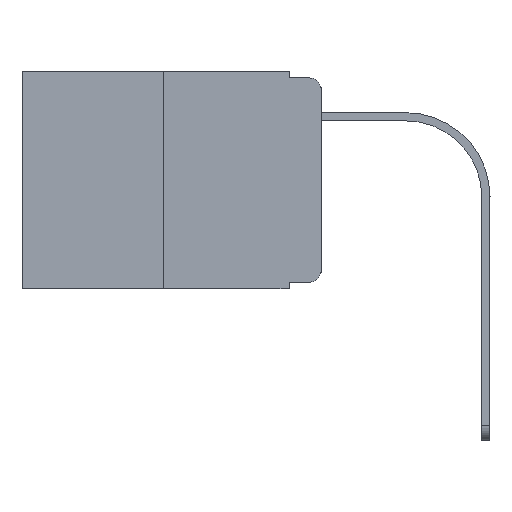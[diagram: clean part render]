
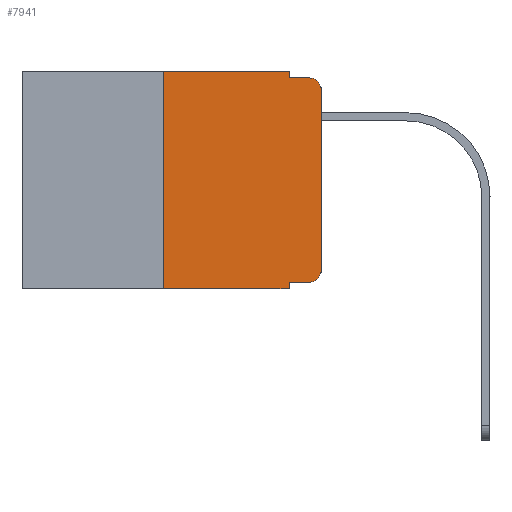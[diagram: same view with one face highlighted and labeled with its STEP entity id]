
A CAD part, left-side view. The second image highlights one B-rep face of the part: STEP entity #7941.
In plain terms, the highlighted planar face has unit normal (-1, 0, 0).
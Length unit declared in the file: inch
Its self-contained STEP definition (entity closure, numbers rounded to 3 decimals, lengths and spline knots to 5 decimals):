
#130 = VECTOR ( 'NONE', #17695, 39.37008 ) ;
#359 = PLANE ( 'NONE',  #10256 ) ;
#586 = DIRECTION ( 'NONE',  ( 0., -1., 0. ) ) ;
#771 = CIRCLE ( 'NONE', #4954, 0.02 ) ;
#1702 = VERTEX_POINT ( 'NONE', #5102 ) ;
#1730 = LINE ( 'NONE', #12129, #6146 ) ;
#1750 = EDGE_CURVE ( 'NONE', #2048, #12423, #1730, .T. ) ;
#1771 = DIRECTION ( 'NONE',  ( 1., 0., 0. ) ) ;
#1846 = VERTEX_POINT ( 'NONE', #15604 ) ;
#2048 = VERTEX_POINT ( 'NONE', #16135 ) ;
#4032 = ORIENTED_EDGE ( 'NONE', *, *, #6118, .T. ) ;
#4189 = CARTESIAN_POINT ( 'NONE',  ( 0., 0.25, -0.343 ) ) ;
#4335 = VECTOR ( 'NONE', #13827, 39.37008 ) ;
#4568 = EDGE_CURVE ( 'NONE', #15227, #15545, #4579, .T. ) ;
#4579 = LINE ( 'NONE', #11180, #130 ) ;
#4929 = ORIENTED_EDGE ( 'NONE', *, *, #4568, .F. ) ;
#4954 = AXIS2_PLACEMENT_3D ( 'NONE', #9097, #15707, #5849 ) ;
#5032 = VERTEX_POINT ( 'NONE', #9274 ) ;
#5056 = EDGE_CURVE ( 'NONE', #1702, #5032, #15770, .T. ) ;
#5102 = CARTESIAN_POINT ( 'NONE',  ( 0., 0.051, -0.333 ) ) ;
#5849 = DIRECTION ( 'NONE',  ( 0., 0., -1. ) ) ;
#6114 = DIRECTION ( 'NONE',  ( -1., 0., 0. ) ) ;
#6118 = EDGE_CURVE ( 'NONE', #1846, #15312, #16435, .T. ) ;
#6146 = VECTOR ( 'NONE', #13327, 39.37008 ) ;
#6446 = ORIENTED_EDGE ( 'NONE', *, *, #16430, .T. ) ;
#6558 = VECTOR ( 'NONE', #8209, 39.37008 ) ;
#6667 = CARTESIAN_POINT ( 'NONE',  ( 0., 0.02, -0.333 ) ) ;
#7365 = EDGE_CURVE ( 'NONE', #15545, #2048, #10957, .T. ) ;
#7546 = CARTESIAN_POINT ( 'NONE',  ( 0., 0.051, 0. ) ) ;
#7941 = ADVANCED_FACE ( 'NONE', ( #11637 ), #359, .F. ) ;
#8165 = ORIENTED_EDGE ( 'NONE', *, *, #1750, .F. ) ;
#8209 = DIRECTION ( 'NONE',  ( 0., 0., 1. ) ) ;
#8402 = DIRECTION ( 'NONE',  ( 0., 0., -1. ) ) ;
#8715 = DIRECTION ( 'NONE',  ( 0., 0., 1. ) ) ;
#9097 = CARTESIAN_POINT ( 'NONE',  ( 0., 0.02, -0.03 ) ) ;
#9264 = DIRECTION ( 'NONE',  ( 0., 0., -1. ) ) ;
#9274 = CARTESIAN_POINT ( 'NONE',  ( 0., 0.051, -0.343 ) ) ;
#9454 = ORIENTED_EDGE ( 'NONE', *, *, #19110, .T. ) ;
#10018 = CARTESIAN_POINT ( 'NONE',  ( 0., 0.473, 0. ) ) ;
#10256 = AXIS2_PLACEMENT_3D ( 'NONE', #10018, #1771, #8402 ) ;
#10433 = CARTESIAN_POINT ( 'NONE',  ( 0., 0.25, 0. ) ) ;
#10926 = AXIS2_PLACEMENT_3D ( 'NONE', #17606, #6114, #9264 ) ;
#10957 = LINE ( 'NONE', #21236, #12675 ) ;
#11180 = CARTESIAN_POINT ( 'NONE',  ( 0., 0.473, 0. ) ) ;
#11637 = FACE_OUTER_BOUND ( 'NONE', #20930, .T. ) ;
#12129 = CARTESIAN_POINT ( 'NONE',  ( 0., 0.051, -0.01 ) ) ;
#12346 = EDGE_CURVE ( 'NONE', #15312, #12423, #771, .T. ) ;
#12412 = VECTOR ( 'NONE', #8715, 39.37008 ) ;
#12423 = VERTEX_POINT ( 'NONE', #17876 ) ;
#12537 = VERTEX_POINT ( 'NONE', #4189 ) ;
#12675 = VECTOR ( 'NONE', #19197, 39.37008 ) ;
#12687 = CARTESIAN_POINT ( 'NONE',  ( 0., 0.25, 0. ) ) ;
#12750 = ORIENTED_EDGE ( 'NONE', *, *, #5056, .F. ) ;
#12808 = EDGE_CURVE ( 'NONE', #12537, #5032, #13512, .T. ) ;
#12925 = VECTOR ( 'NONE', #586, 39.37008 ) ;
#12974 = LINE ( 'NONE', #19597, #16541 ) ;
#13327 = DIRECTION ( 'NONE',  ( 0., -1., 0. ) ) ;
#13512 = LINE ( 'NONE', #16654, #12925 ) ;
#13827 = DIRECTION ( 'NONE',  ( 0., 0., -1. ) ) ;
#14706 = DIRECTION ( 'NONE',  ( 0., -1., 0. ) ) ;
#14739 = ORIENTED_EDGE ( 'NONE', *, *, #12346, .T. ) ;
#15227 = VERTEX_POINT ( 'NONE', #12687 ) ;
#15312 = VERTEX_POINT ( 'NONE', #18203 ) ;
#15545 = VERTEX_POINT ( 'NONE', #20683 ) ;
#15604 = CARTESIAN_POINT ( 'NONE',  ( 0., 0., -0.313 ) ) ;
#15707 = DIRECTION ( 'NONE',  ( -1., 0., 0. ) ) ;
#15770 = LINE ( 'NONE', #7546, #4335 ) ;
#15920 = ORIENTED_EDGE ( 'NONE', *, *, #7365, .F. ) ;
#16135 = CARTESIAN_POINT ( 'NONE',  ( 0., 0.051, -0.01 ) ) ;
#16430 = EDGE_CURVE ( 'NONE', #20606, #1846, #16799, .T. ) ;
#16435 = LINE ( 'NONE', #21108, #6558 ) ;
#16541 = VECTOR ( 'NONE', #14706, 39.37008 ) ;
#16654 = CARTESIAN_POINT ( 'NONE',  ( 0., 0.473, -0.343 ) ) ;
#16799 = CIRCLE ( 'NONE', #10926, 0.02 ) ;
#17606 = CARTESIAN_POINT ( 'NONE',  ( 0., 0.02, -0.313 ) ) ;
#17695 = DIRECTION ( 'NONE',  ( 0., -1., 0. ) ) ;
#17876 = CARTESIAN_POINT ( 'NONE',  ( 0., 0.02, -0.01 ) ) ;
#17932 = ORIENTED_EDGE ( 'NONE', *, *, #12808, .T. ) ;
#18203 = CARTESIAN_POINT ( 'NONE',  ( 0., 0., -0.03 ) ) ;
#18575 = LINE ( 'NONE', #10433, #12412 ) ;
#19110 = EDGE_CURVE ( 'NONE', #1702, #20606, #12974, .T. ) ;
#19197 = DIRECTION ( 'NONE',  ( 0., 0., -1. ) ) ;
#19426 = ORIENTED_EDGE ( 'NONE', *, *, #19610, .F. ) ;
#19597 = CARTESIAN_POINT ( 'NONE',  ( 0., 0.051, -0.333 ) ) ;
#19610 = EDGE_CURVE ( 'NONE', #12537, #15227, #18575, .T. ) ;
#20606 = VERTEX_POINT ( 'NONE', #6667 ) ;
#20683 = CARTESIAN_POINT ( 'NONE',  ( 0., 0.051, 0. ) ) ;
#20930 = EDGE_LOOP ( 'NONE', ( #4032, #14739, #8165, #15920, #4929, #19426, #17932, #12750, #9454, #6446 ) ) ;
#21108 = CARTESIAN_POINT ( 'NONE',  ( 0., 0., 0. ) ) ;
#21236 = CARTESIAN_POINT ( 'NONE',  ( 0., 0.051, 0. ) ) ;
